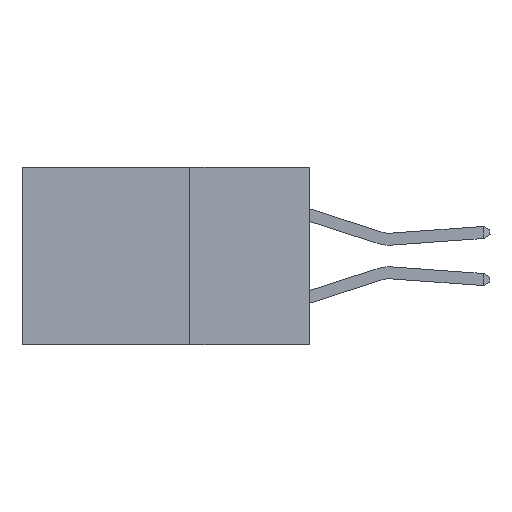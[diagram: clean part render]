
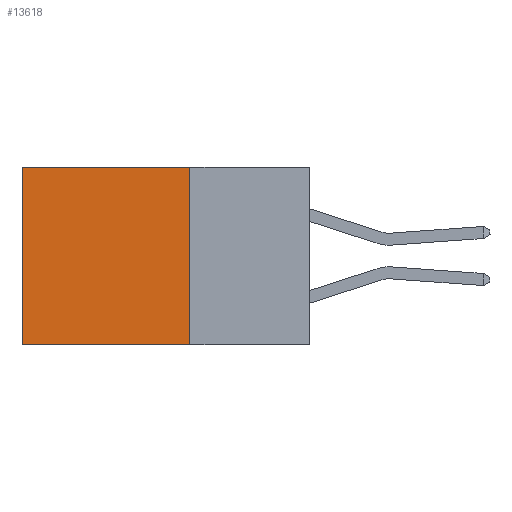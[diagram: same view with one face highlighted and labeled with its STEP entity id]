
A CAD part, left-side view. The second image highlights one B-rep face of the part: STEP entity #13618.
In plain terms, the highlighted planar face has unit normal (-1, 0, 0).
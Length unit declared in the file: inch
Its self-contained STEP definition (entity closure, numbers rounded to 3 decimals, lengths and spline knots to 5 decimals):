
#378 = DIRECTION ( 'NONE',  ( 0., 1., 0. ) ) ;
#495 = VECTOR ( 'NONE', #1403, 39.37008 ) ;
#680 = CARTESIAN_POINT ( 'NONE',  ( 0.2615, 0.25, 0. ) ) ;
#1294 = CARTESIAN_POINT ( 'NONE',  ( 0.2615, 0.25, -0.37 ) ) ;
#1386 = CARTESIAN_POINT ( 'NONE',  ( 0.2615, 0.6, -0.37 ) ) ;
#1403 = DIRECTION ( 'NONE',  ( 0., 0., -1. ) ) ;
#1771 = ORIENTED_EDGE ( 'NONE', *, *, #12031, .F. ) ;
#1790 = ORIENTED_EDGE ( 'NONE', *, *, #1969, .F. ) ;
#1858 = CARTESIAN_POINT ( 'NONE',  ( 0.2615, 0.6, 0. ) ) ;
#1969 = EDGE_CURVE ( 'NONE', #7030, #2945, #2459, .T. ) ;
#2415 = LINE ( 'NONE', #2774, #8036 ) ;
#2453 = EDGE_CURVE ( 'NONE', #13324, #11444, #8761, .T. ) ;
#2459 = LINE ( 'NONE', #5766, #8082 ) ;
#2464 = DIRECTION ( 'NONE',  ( 0., 0., -1. ) ) ;
#2553 = EDGE_CURVE ( 'NONE', #7030, #13324, #10313, .T. ) ;
#2774 = CARTESIAN_POINT ( 'NONE',  ( 0.2615, 0.25, -0.37 ) ) ;
#2818 = CARTESIAN_POINT ( 'NONE',  ( 0.2615, 0.25, 0. ) ) ;
#2936 = CARTESIAN_POINT ( 'NONE',  ( 0.2615, 0.6, -0.37 ) ) ;
#2945 = VERTEX_POINT ( 'NONE', #6157 ) ;
#5766 = CARTESIAN_POINT ( 'NONE',  ( 0.2615, 0.25, -0.37 ) ) ;
#6035 = DIRECTION ( 'NONE',  ( 0., 0., -1. ) ) ;
#6157 = CARTESIAN_POINT ( 'NONE',  ( 0.2615, 0.25, -0.37 ) ) ;
#6371 = AXIS2_PLACEMENT_3D ( 'NONE', #1294, #9158, #2464 ) ;
#7011 = VECTOR ( 'NONE', #378, 39.37008 ) ;
#7030 = VERTEX_POINT ( 'NONE', #2818 ) ;
#7255 = DIRECTION ( 'NONE',  ( 0., 1., 0. ) ) ;
#8036 = VECTOR ( 'NONE', #7255, 39.37008 ) ;
#8082 = VECTOR ( 'NONE', #6035, 39.37008 ) ;
#8123 = ORIENTED_EDGE ( 'NONE', *, *, #2453, .T. ) ;
#8761 = LINE ( 'NONE', #1386, #495 ) ;
#9118 = PLANE ( 'NONE',  #6371 ) ;
#9158 = DIRECTION ( 'NONE',  ( 1., 0., 0. ) ) ;
#10313 = LINE ( 'NONE', #680, #7011 ) ;
#10662 = ORIENTED_EDGE ( 'NONE', *, *, #2553, .T. ) ;
#11444 = VERTEX_POINT ( 'NONE', #2936 ) ;
#12031 = EDGE_CURVE ( 'NONE', #2945, #11444, #2415, .T. ) ;
#12292 = FACE_OUTER_BOUND ( 'NONE', #12412, .T. ) ;
#12412 = EDGE_LOOP ( 'NONE', ( #8123, #1771, #1790, #10662 ) ) ;
#13324 = VERTEX_POINT ( 'NONE', #1858 ) ;
#13618 = ADVANCED_FACE ( 'NONE', ( #12292 ), #9118, .F. ) ;
